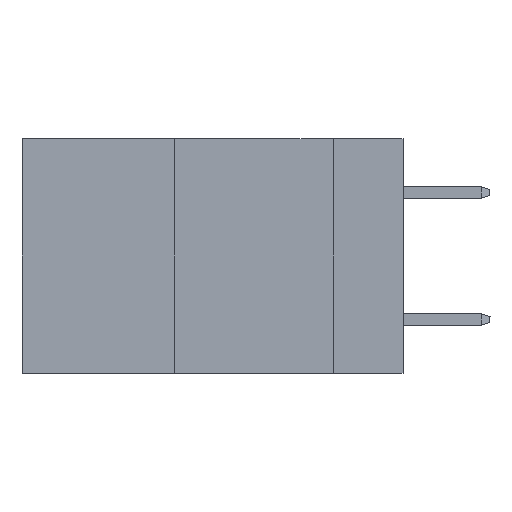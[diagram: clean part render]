
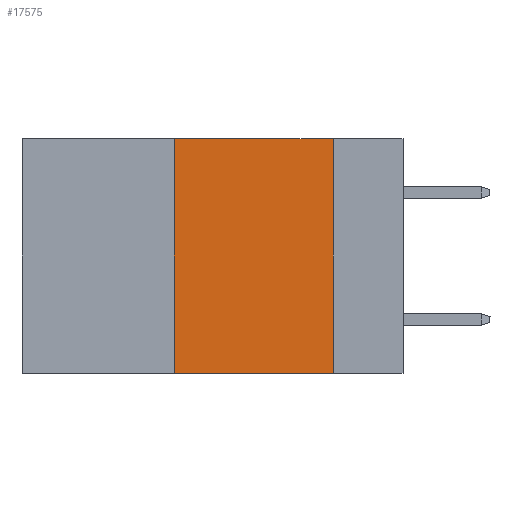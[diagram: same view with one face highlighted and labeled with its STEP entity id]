
A CAD part, left-side view. The second image highlights one B-rep face of the part: STEP entity #17575.
In plain terms, the highlighted planar face has unit normal (-1, 0, 0).
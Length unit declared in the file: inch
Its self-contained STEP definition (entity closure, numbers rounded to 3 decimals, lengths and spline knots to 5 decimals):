
#1287 = CARTESIAN_POINT ( 'NONE',  ( 0., 0.6, 0. ) ) ;
#3542 = DIRECTION ( 'NONE',  ( 1., 0., 0. ) ) ;
#3714 = EDGE_LOOP ( 'NONE', ( #8253, #28414, #19499, #12842 ) ) ;
#4030 = LINE ( 'NONE', #13486, #28982 ) ;
#5394 = VERTEX_POINT ( 'NONE', #16699 ) ;
#7525 = AXIS2_PLACEMENT_3D ( 'NONE', #19647, #3542, #15009 ) ;
#8253 = ORIENTED_EDGE ( 'NONE', *, *, #22105, .F. ) ;
#10566 = LINE ( 'NONE', #1287, #22306 ) ;
#11160 = EDGE_CURVE ( 'NONE', #26642, #18448, #11816, .T. ) ;
#11324 = EDGE_CURVE ( 'NONE', #18448, #23785, #10566, .T. ) ;
#11816 = LINE ( 'NONE', #21249, #21335 ) ;
#12842 = ORIENTED_EDGE ( 'NONE', *, *, #29927, .T. ) ;
#13486 = CARTESIAN_POINT ( 'NONE',  ( 0., 0.11, 0. ) ) ;
#15009 = DIRECTION ( 'NONE',  ( 0., 0., -1. ) ) ;
#15736 = CARTESIAN_POINT ( 'NONE',  ( 0., 0.36, -0.37 ) ) ;
#16699 = CARTESIAN_POINT ( 'NONE',  ( 0., 0.11, -0.37 ) ) ;
#17575 = ADVANCED_FACE ( 'NONE', ( #21802 ), #26684, .F. ) ;
#18448 = VERTEX_POINT ( 'NONE', #24908 ) ;
#19465 = LINE ( 'NONE', #19612, #24321 ) ;
#19499 = ORIENTED_EDGE ( 'NONE', *, *, #11160, .F. ) ;
#19612 = CARTESIAN_POINT ( 'NONE',  ( 0., 0.6, -0.37 ) ) ;
#19647 = CARTESIAN_POINT ( 'NONE',  ( 0., 0.6, 0. ) ) ;
#20874 = DIRECTION ( 'NONE',  ( 0., 0., -1. ) ) ;
#21249 = CARTESIAN_POINT ( 'NONE',  ( 0., 0.36, 0. ) ) ;
#21335 = VECTOR ( 'NONE', #28000, 39.37008 ) ;
#21523 = CARTESIAN_POINT ( 'NONE',  ( 0., 0.11, 0. ) ) ;
#21802 = FACE_OUTER_BOUND ( 'NONE', #3714, .T. ) ;
#22105 = EDGE_CURVE ( 'NONE', #23785, #5394, #4030, .T. ) ;
#22306 = VECTOR ( 'NONE', #27054, 39.37008 ) ;
#23785 = VERTEX_POINT ( 'NONE', #21523 ) ;
#24321 = VECTOR ( 'NONE', #28354, 39.37008 ) ;
#24908 = CARTESIAN_POINT ( 'NONE',  ( 0., 0.36, 0. ) ) ;
#26642 = VERTEX_POINT ( 'NONE', #15736 ) ;
#26684 = PLANE ( 'NONE',  #7525 ) ;
#27054 = DIRECTION ( 'NONE',  ( 0., -1., 0. ) ) ;
#28000 = DIRECTION ( 'NONE',  ( 0., 0., 1. ) ) ;
#28354 = DIRECTION ( 'NONE',  ( 0., -1., 0. ) ) ;
#28414 = ORIENTED_EDGE ( 'NONE', *, *, #11324, .F. ) ;
#28982 = VECTOR ( 'NONE', #20874, 39.37008 ) ;
#29927 = EDGE_CURVE ( 'NONE', #26642, #5394, #19465, .T. ) ;
